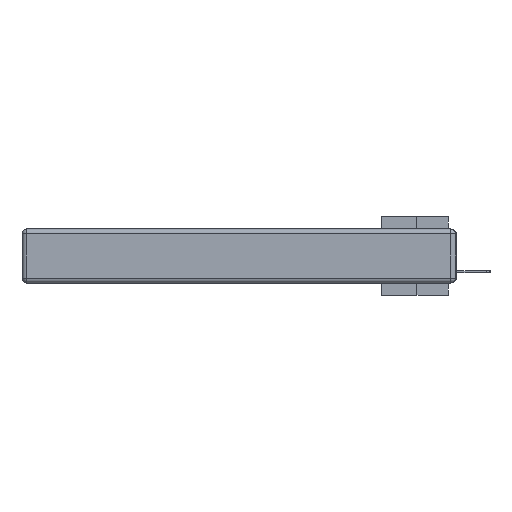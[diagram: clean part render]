
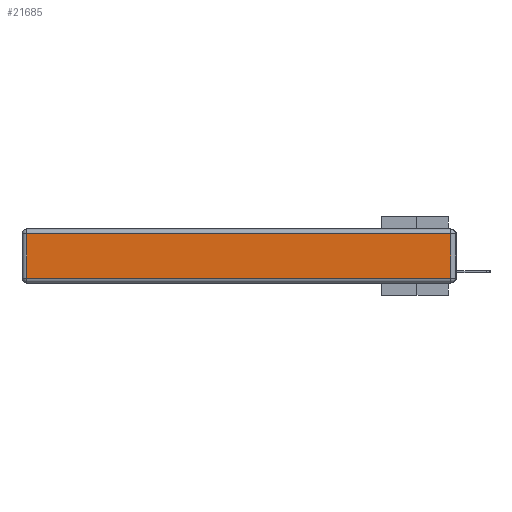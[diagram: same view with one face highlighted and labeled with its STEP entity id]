
A CAD part, left-side view. The second image highlights one B-rep face of the part: STEP entity #21685.
In plain terms, the highlighted planar face has unit normal (-1, 0, 0).
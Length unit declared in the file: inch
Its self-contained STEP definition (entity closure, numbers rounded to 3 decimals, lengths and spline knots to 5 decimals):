
#1173 = ORIENTED_EDGE ( 'NONE', *, *, #6704, .T. ) ;
#1562 = EDGE_CURVE ( 'NONE', #33843, #31189, #27965, .T. ) ;
#2099 = DIRECTION ( 'NONE',  ( -1., 0., 0. ) ) ;
#2266 = ORIENTED_EDGE ( 'NONE', *, *, #27870, .T. ) ;
#2324 = CARTESIAN_POINT ( 'NONE',  ( 0., 0., -0.343 ) ) ;
#2411 = VERTEX_POINT ( 'NONE', #20168 ) ;
#4591 = DIRECTION ( 'NONE',  ( 0., 1., 0. ) ) ;
#5002 = EDGE_LOOP ( 'NONE', ( #15118, #2266, #1173, #8594 ) ) ;
#5582 = VECTOR ( 'NONE', #31219, 39.37008 ) ;
#5992 = LINE ( 'NONE', #27094, #21752 ) ;
#6483 = FACE_OUTER_BOUND ( 'NONE', #5002, .T. ) ;
#6704 = EDGE_CURVE ( 'NONE', #11381, #2411, #25565, .T. ) ;
#8594 = ORIENTED_EDGE ( 'NONE', *, *, #26289, .T. ) ;
#10074 = CARTESIAN_POINT ( 'NONE',  ( 0., 0., -0.313 ) ) ;
#10726 = DIRECTION ( 'NONE',  ( 0., 0., -1. ) ) ;
#11381 = VERTEX_POINT ( 'NONE', #31702 ) ;
#12854 = PLANE ( 'NONE',  #16809 ) ;
#14106 = DIRECTION ( 'NONE',  ( 0., 0., 1. ) ) ;
#15118 = ORIENTED_EDGE ( 'NONE', *, *, #1562, .T. ) ;
#15743 = DIRECTION ( 'NONE',  ( 0., 0., 1. ) ) ;
#16809 = AXIS2_PLACEMENT_3D ( 'NONE', #2324, #2099, #15743 ) ;
#20168 = CARTESIAN_POINT ( 'NONE',  ( 0., 2.72, -0.03 ) ) ;
#21685 = ADVANCED_FACE ( 'NONE', ( #6483 ), #12854, .T. ) ;
#21752 = VECTOR ( 'NONE', #14106, 39.37008 ) ;
#22237 = VECTOR ( 'NONE', #4591, 39.37008 ) ;
#22646 = CARTESIAN_POINT ( 'NONE',  ( 0., 2.72, -0.313 ) ) ;
#25565 = LINE ( 'NONE', #26014, #22237 ) ;
#26014 = CARTESIAN_POINT ( 'NONE',  ( 0., 2.75, -0.03 ) ) ;
#26289 = EDGE_CURVE ( 'NONE', #2411, #33843, #32628, .T. ) ;
#26304 = CARTESIAN_POINT ( 'NONE',  ( 0., 2.72, -0.343 ) ) ;
#27094 = CARTESIAN_POINT ( 'NONE',  ( 0., 0.03, -0.343 ) ) ;
#27870 = EDGE_CURVE ( 'NONE', #31189, #11381, #5992, .T. ) ;
#27965 = LINE ( 'NONE', #10074, #5582 ) ;
#29460 = CARTESIAN_POINT ( 'NONE',  ( 0., 0.03, -0.313 ) ) ;
#30181 = VECTOR ( 'NONE', #10726, 39.37008 ) ;
#31189 = VERTEX_POINT ( 'NONE', #29460 ) ;
#31219 = DIRECTION ( 'NONE',  ( 0., -1., 0. ) ) ;
#31702 = CARTESIAN_POINT ( 'NONE',  ( 0., 0.03, -0.03 ) ) ;
#32628 = LINE ( 'NONE', #26304, #30181 ) ;
#33843 = VERTEX_POINT ( 'NONE', #22646 ) ;
